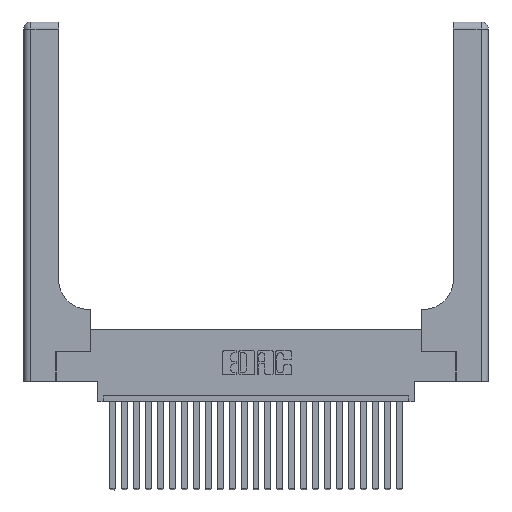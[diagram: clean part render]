
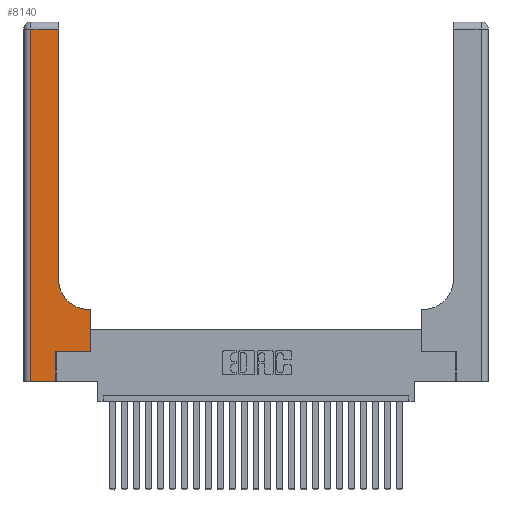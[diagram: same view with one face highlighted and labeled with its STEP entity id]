
A CAD part, top view. The second image highlights one B-rep face of the part: STEP entity #8140.
In plain terms, the highlighted planar face has unit normal (0, 0, 1).
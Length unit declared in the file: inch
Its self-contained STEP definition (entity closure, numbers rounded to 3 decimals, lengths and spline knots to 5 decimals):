
#26 = CARTESIAN_POINT ( 'NONE',  ( 0.5415, 0.6, 0.37 ) ) ;
#84 = VECTOR ( 'NONE', #3116, 39.37008 ) ;
#552 = VERTEX_POINT ( 'NONE', #26 ) ;
#1121 = CARTESIAN_POINT ( 'NONE',  ( 0.5585, 0.25, 0.37 ) ) ;
#1194 = CARTESIAN_POINT ( 'NONE',  ( 0.269, 0., 0.37 ) ) ;
#1403 = CARTESIAN_POINT ( 'NONE',  ( 0., 0., 0.37 ) ) ;
#1492 = ORIENTED_EDGE ( 'NONE', *, *, #17269, .T. ) ;
#3039 = VERTEX_POINT ( 'NONE', #3292 ) ;
#3116 = DIRECTION ( 'NONE',  ( 0., -1., 0. ) ) ;
#3292 = CARTESIAN_POINT ( 'NONE',  ( 0.06, 2.94, 0.37 ) ) ;
#3463 = EDGE_CURVE ( 'NONE', #552, #8810, #9776, .T. ) ;
#5276 = EDGE_CURVE ( 'NONE', #7139, #552, #16617, .T. ) ;
#5793 = PLANE ( 'NONE',  #19948 ) ;
#6224 = DIRECTION ( 'NONE',  ( 0., 0., -1. ) ) ;
#6586 = CARTESIAN_POINT ( 'NONE',  ( 0.5415, 0.85, 0.37 ) ) ;
#7139 = VERTEX_POINT ( 'NONE', #14719 ) ;
#7410 = DIRECTION ( 'NONE',  ( 1., 0., 0. ) ) ;
#7764 = DIRECTION ( 'NONE',  ( 0., 0., -1. ) ) ;
#7807 = ORIENTED_EDGE ( 'NONE', *, *, #13572, .T. ) ;
#8140 = ADVANCED_FACE ( 'NONE', ( #9223 ), #5793, .F. ) ;
#8446 = EDGE_CURVE ( 'NONE', #20076, #22581, #21781, .T. ) ;
#8810 = VERTEX_POINT ( 'NONE', #14001 ) ;
#8869 = CARTESIAN_POINT ( 'NONE',  ( 0.5585, 0.25, 0.37 ) ) ;
#9223 = FACE_OUTER_BOUND ( 'NONE', #11270, .T. ) ;
#9408 = DIRECTION ( 'NONE',  ( 1., 0., 0. ) ) ;
#9776 = CIRCLE ( 'NONE', #15642, 0.25 ) ;
#10498 = VECTOR ( 'NONE', #15204, 39.37008 ) ;
#10590 = ORIENTED_EDGE ( 'NONE', *, *, #25127, .T. ) ;
#10750 = ORIENTED_EDGE ( 'NONE', *, *, #17684, .T. ) ;
#11270 = EDGE_LOOP ( 'NONE', ( #24344, #10590, #20055, #1492, #25895, #7807, #10750, #22737, #21017 ) ) ;
#11459 = LINE ( 'NONE', #1403, #24695 ) ;
#12002 = CARTESIAN_POINT ( 'NONE',  ( 0.2915, 3., 0.37 ) ) ;
#12327 = DIRECTION ( 'NONE',  ( 1., 0., 0. ) ) ;
#12538 = CARTESIAN_POINT ( 'NONE',  ( 0.2915, 2.94, 0.37 ) ) ;
#13130 = VERTEX_POINT ( 'NONE', #12538 ) ;
#13572 = EDGE_CURVE ( 'NONE', #22581, #16385, #22647, .T. ) ;
#14001 = CARTESIAN_POINT ( 'NONE',  ( 0.2915, 0.85, 0.37 ) ) ;
#14715 = VECTOR ( 'NONE', #16802, 39.37008 ) ;
#14719 = CARTESIAN_POINT ( 'NONE',  ( 0.5585, 0.6, 0.37 ) ) ;
#14834 = VECTOR ( 'NONE', #17207, 39.37008 ) ;
#14920 = CARTESIAN_POINT ( 'NONE',  ( 0.269, 0., 0.37 ) ) ;
#15204 = DIRECTION ( 'NONE',  ( 0., 1., 0. ) ) ;
#15642 = AXIS2_PLACEMENT_3D ( 'NONE', #6586, #6224, #12327 ) ;
#16093 = CARTESIAN_POINT ( 'NONE',  ( 0.2915, 0.6, 0.37 ) ) ;
#16385 = VERTEX_POINT ( 'NONE', #8869 ) ;
#16617 = LINE ( 'NONE', #16093, #16937 ) ;
#16802 = DIRECTION ( 'NONE',  ( -1., 0., 0. ) ) ;
#16937 = VECTOR ( 'NONE', #20157, 39.37008 ) ;
#17207 = DIRECTION ( 'NONE',  ( 0., 1., 0. ) ) ;
#17269 = EDGE_CURVE ( 'NONE', #19651, #20076, #11459, .T. ) ;
#17638 = CARTESIAN_POINT ( 'NONE',  ( 0.269, 0.25, 0.37 ) ) ;
#17684 = EDGE_CURVE ( 'NONE', #16385, #7139, #25601, .T. ) ;
#18926 = CARTESIAN_POINT ( 'NONE',  ( 0.06, 3., 0.37 ) ) ;
#19355 = CARTESIAN_POINT ( 'NONE',  ( 0.269, 0.25, 0.37 ) ) ;
#19651 = VERTEX_POINT ( 'NONE', #20299 ) ;
#19948 = AXIS2_PLACEMENT_3D ( 'NONE', #25724, #7764, #21936 ) ;
#20055 = ORIENTED_EDGE ( 'NONE', *, *, #25213, .T. ) ;
#20076 = VERTEX_POINT ( 'NONE', #14920 ) ;
#20123 = VECTOR ( 'NONE', #9408, 39.37008 ) ;
#20157 = DIRECTION ( 'NONE',  ( -1., 0., 0. ) ) ;
#20299 = CARTESIAN_POINT ( 'NONE',  ( 0.06, 0., 0.37 ) ) ;
#21017 = ORIENTED_EDGE ( 'NONE', *, *, #3463, .T. ) ;
#21162 = VECTOR ( 'NONE', #24067, 39.37008 ) ;
#21781 = LINE ( 'NONE', #1194, #14834 ) ;
#21791 = EDGE_CURVE ( 'NONE', #8810, #13130, #25596, .T. ) ;
#21936 = DIRECTION ( 'NONE',  ( -1., 0., 0. ) ) ;
#22581 = VERTEX_POINT ( 'NONE', #19355 ) ;
#22647 = LINE ( 'NONE', #17638, #20123 ) ;
#22737 = ORIENTED_EDGE ( 'NONE', *, *, #5276, .T. ) ;
#24067 = DIRECTION ( 'NONE',  ( 0., 1., 0. ) ) ;
#24344 = ORIENTED_EDGE ( 'NONE', *, *, #21791, .T. ) ;
#24695 = VECTOR ( 'NONE', #7410, 39.37008 ) ;
#24741 = CARTESIAN_POINT ( 'NONE',  ( 0., 2.94, 0.37 ) ) ;
#24811 = LINE ( 'NONE', #24741, #14715 ) ;
#25126 = LINE ( 'NONE', #18926, #84 ) ;
#25127 = EDGE_CURVE ( 'NONE', #13130, #3039, #24811, .T. ) ;
#25213 = EDGE_CURVE ( 'NONE', #3039, #19651, #25126, .T. ) ;
#25596 = LINE ( 'NONE', #12002, #21162 ) ;
#25601 = LINE ( 'NONE', #1121, #10498 ) ;
#25724 = CARTESIAN_POINT ( 'NONE',  ( 0., 3., 0.37 ) ) ;
#25895 = ORIENTED_EDGE ( 'NONE', *, *, #8446, .T. ) ;
